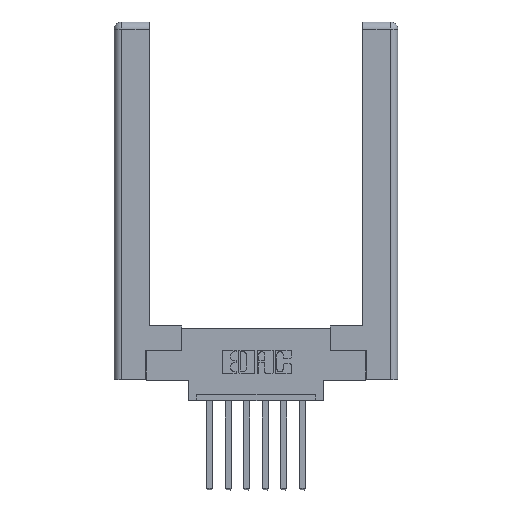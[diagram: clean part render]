
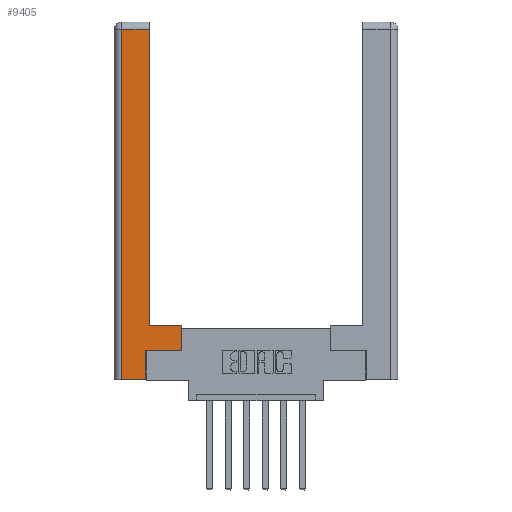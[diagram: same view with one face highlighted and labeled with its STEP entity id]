
A CAD part, top view. The second image highlights one B-rep face of the part: STEP entity #9405.
In plain terms, the highlighted planar face has unit normal (0, 0, 1).
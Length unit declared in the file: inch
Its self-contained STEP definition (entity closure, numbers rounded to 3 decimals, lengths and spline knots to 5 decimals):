
#14 = LINE ( 'NONE', #639, #4136 ) ;
#49 = EDGE_CURVE ( 'NONE', #10468, #7575, #3699, .T. ) ;
#297 = CARTESIAN_POINT ( 'NONE',  ( 0., 0., 0. ) ) ;
#331 = VERTEX_POINT ( 'NONE', #2233 ) ;
#639 = CARTESIAN_POINT ( 'NONE',  ( 0.295, 3., 0. ) ) ;
#707 = ORIENTED_EDGE ( 'NONE', *, *, #4270, .T. ) ;
#865 = VECTOR ( 'NONE', #7205, 39.37008 ) ;
#909 = VECTOR ( 'NONE', #6790, 39.37008 ) ;
#1154 = DIRECTION ( 'NONE',  ( -1., 0., 0. ) ) ;
#1172 = CARTESIAN_POINT ( 'NONE',  ( 0.265, 0., 0. ) ) ;
#1182 = VERTEX_POINT ( 'NONE', #1697 ) ;
#1427 = CARTESIAN_POINT ( 'NONE',  ( 0.565, 0.45, 0. ) ) ;
#1442 = VECTOR ( 'NONE', #9045, 39.37008 ) ;
#1697 = CARTESIAN_POINT ( 'NONE',  ( 0.295, 0.45, 0. ) ) ;
#2096 = DIRECTION ( 'NONE',  ( 0., 1., 0. ) ) ;
#2233 = CARTESIAN_POINT ( 'NONE',  ( 0.0615, 2.94, 0. ) ) ;
#2263 = VECTOR ( 'NONE', #3683, 39.37008 ) ;
#2733 = LINE ( 'NONE', #3607, #1442 ) ;
#2884 = ORIENTED_EDGE ( 'NONE', *, *, #49, .T. ) ;
#2990 = CARTESIAN_POINT ( 'NONE',  ( 0.265, 0.245, 0. ) ) ;
#3115 = AXIS2_PLACEMENT_3D ( 'NONE', #297, #3917, #1154 ) ;
#3219 = LINE ( 'NONE', #4182, #10406 ) ;
#3607 = CARTESIAN_POINT ( 'NONE',  ( 0.565, 0.245, 0. ) ) ;
#3683 = DIRECTION ( 'NONE',  ( 0., 1., 0. ) ) ;
#3699 = LINE ( 'NONE', #8214, #2263 ) ;
#3872 = VECTOR ( 'NONE', #2096, 39.37008 ) ;
#3917 = DIRECTION ( 'NONE',  ( 0., 0., -1. ) ) ;
#4136 = VECTOR ( 'NONE', #9104, 39.37008 ) ;
#4182 = CARTESIAN_POINT ( 'NONE',  ( 0.0615, 2.94, 0. ) ) ;
#4270 = EDGE_CURVE ( 'NONE', #5095, #11459, #6269, .T. ) ;
#4279 = DIRECTION ( 'NONE',  ( -1., 0., 0. ) ) ;
#4297 = ORIENTED_EDGE ( 'NONE', *, *, #11673, .T. ) ;
#4808 = DIRECTION ( 'NONE',  ( -1., 0., 0. ) ) ;
#4831 = EDGE_CURVE ( 'NONE', #11459, #7058, #10771, .T. ) ;
#5095 = VERTEX_POINT ( 'NONE', #10647 ) ;
#5122 = EDGE_CURVE ( 'NONE', #1182, #5632, #14, .T. ) ;
#5158 = FACE_OUTER_BOUND ( 'NONE', #6509, .T. ) ;
#5632 = VERTEX_POINT ( 'NONE', #11142 ) ;
#6167 = ORIENTED_EDGE ( 'NONE', *, *, #10449, .T. ) ;
#6269 = LINE ( 'NONE', #8918, #865 ) ;
#6509 = EDGE_LOOP ( 'NONE', ( #7080, #7902, #7504, #707, #6981, #6167, #2884, #4297 ) ) ;
#6790 = DIRECTION ( 'NONE',  ( 0., -1., 0. ) ) ;
#6981 = ORIENTED_EDGE ( 'NONE', *, *, #4831, .T. ) ;
#7028 = CARTESIAN_POINT ( 'NONE',  ( 0.265, 0.245, 0. ) ) ;
#7058 = VERTEX_POINT ( 'NONE', #7028 ) ;
#7080 = ORIENTED_EDGE ( 'NONE', *, *, #5122, .T. ) ;
#7205 = DIRECTION ( 'NONE',  ( 1., 0., 0. ) ) ;
#7504 = ORIENTED_EDGE ( 'NONE', *, *, #9147, .T. ) ;
#7575 = VERTEX_POINT ( 'NONE', #1427 ) ;
#7589 = PLANE ( 'NONE',  #3115 ) ;
#7631 = CARTESIAN_POINT ( 'NONE',  ( 0.0615, 0., 0. ) ) ;
#7902 = ORIENTED_EDGE ( 'NONE', *, *, #8872, .T. ) ;
#8214 = CARTESIAN_POINT ( 'NONE',  ( 0.565, 0.45, 0. ) ) ;
#8854 = LINE ( 'NONE', #11335, #11551 ) ;
#8872 = EDGE_CURVE ( 'NONE', #5632, #331, #3219, .T. ) ;
#8918 = CARTESIAN_POINT ( 'NONE',  ( 0.265, 0., 0. ) ) ;
#9045 = DIRECTION ( 'NONE',  ( 1., 0., 0. ) ) ;
#9104 = DIRECTION ( 'NONE',  ( 0., 1., 0. ) ) ;
#9147 = EDGE_CURVE ( 'NONE', #331, #5095, #9965, .T. ) ;
#9405 = ADVANCED_FACE ( 'NONE', ( #5158 ), #7589, .F. ) ;
#9965 = LINE ( 'NONE', #7631, #909 ) ;
#10406 = VECTOR ( 'NONE', #4808, 39.37008 ) ;
#10449 = EDGE_CURVE ( 'NONE', #7058, #10468, #2733, .T. ) ;
#10468 = VERTEX_POINT ( 'NONE', #10873 ) ;
#10647 = CARTESIAN_POINT ( 'NONE',  ( 0.0615, 0., 0. ) ) ;
#10771 = LINE ( 'NONE', #2990, #3872 ) ;
#10873 = CARTESIAN_POINT ( 'NONE',  ( 0.565, 0.245, 0. ) ) ;
#11142 = CARTESIAN_POINT ( 'NONE',  ( 0.295, 2.94, 0. ) ) ;
#11335 = CARTESIAN_POINT ( 'NONE',  ( 0.295, 0.45, 0. ) ) ;
#11459 = VERTEX_POINT ( 'NONE', #1172 ) ;
#11551 = VECTOR ( 'NONE', #4279, 39.37008 ) ;
#11673 = EDGE_CURVE ( 'NONE', #7575, #1182, #8854, .T. ) ;
